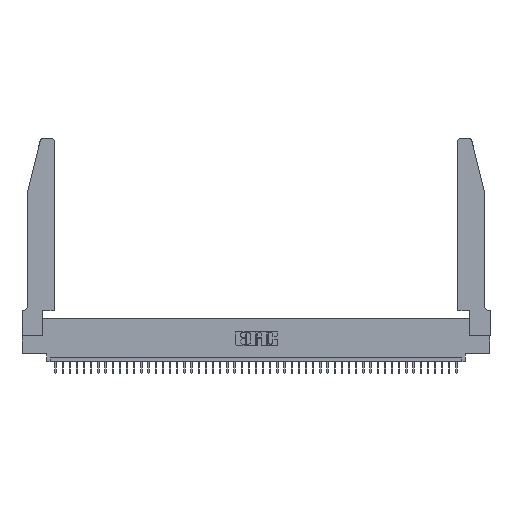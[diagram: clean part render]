
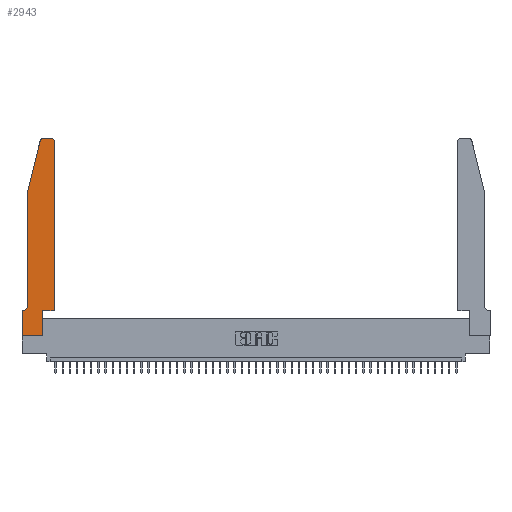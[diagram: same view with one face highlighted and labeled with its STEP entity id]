
A CAD part, top view. The second image highlights one B-rep face of the part: STEP entity #2943.
In plain terms, the highlighted planar face has unit normal (0, 0, 1).
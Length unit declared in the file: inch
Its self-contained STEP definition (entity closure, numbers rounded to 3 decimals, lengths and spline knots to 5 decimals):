
#106 = EDGE_CURVE ( 'NONE', #34860, #22482, #16023, .T. ) ;
#476 = VERTEX_POINT ( 'NONE', #846 ) ;
#504 = CARTESIAN_POINT ( 'NONE',  ( 0.0055, 0.35, 0.37 ) ) ;
#836 = DIRECTION ( 'NONE',  ( 0., 1., 0. ) ) ;
#846 = CARTESIAN_POINT ( 'NONE',  ( 0.4505, 0.35, 0.37 ) ) ;
#949 = LINE ( 'NONE', #4083, #23601 ) ;
#1282 = DIRECTION ( 'NONE',  ( 1., 0., 0. ) ) ;
#1801 = CIRCLE ( 'NONE', #14285, 0.03 ) ;
#1964 = VECTOR ( 'NONE', #4756, 39.37008 ) ;
#2101 = CARTESIAN_POINT ( 'NONE',  ( 0.284, 2.75, 0.37 ) ) ;
#2395 = ORIENTED_EDGE ( 'NONE', *, *, #23045, .T. ) ;
#2943 = ADVANCED_FACE ( 'NONE', ( #12163 ), #3575, .T. ) ;
#3575 = PLANE ( 'NONE',  #34172 ) ;
#4044 = VERTEX_POINT ( 'NONE', #26519 ) ;
#4083 = CARTESIAN_POINT ( 'NONE',  ( 0.4505, 0.35, 0.37 ) ) ;
#4433 = CARTESIAN_POINT ( 'NONE',  ( 0.284, 2.72, 0.37 ) ) ;
#4756 = DIRECTION ( 'NONE',  ( -0.239, -0.971, 0. ) ) ;
#5907 = ORIENTED_EDGE ( 'NONE', *, *, #36275, .T. ) ;
#6338 = VERTEX_POINT ( 'NONE', #42171 ) ;
#6488 = DIRECTION ( 'NONE',  ( -1., 0., 0. ) ) ;
#6923 = CARTESIAN_POINT ( 'NONE',  ( 0., 0., 0.37 ) ) ;
#8188 = EDGE_CURVE ( 'NONE', #476, #33832, #12763, .T. ) ;
#8206 = CARTESIAN_POINT ( 'NONE',  ( 0.2865, 0.35, 0.37 ) ) ;
#9088 = VECTOR ( 'NONE', #36396, 39.37008 ) ;
#9766 = VECTOR ( 'NONE', #41715, 39.37008 ) ;
#11070 = CARTESIAN_POINT ( 'NONE',  ( 0.4205, 2.75, 0.37 ) ) ;
#11316 = VERTEX_POINT ( 'NONE', #11070 ) ;
#11942 = VERTEX_POINT ( 'NONE', #45766 ) ;
#12163 = FACE_OUTER_BOUND ( 'NONE', #22378, .T. ) ;
#12361 = VECTOR ( 'NONE', #15133, 39.37008 ) ;
#12508 = DIRECTION ( 'NONE',  ( 0., 0., -1. ) ) ;
#12763 = LINE ( 'NONE', #30459, #39845 ) ;
#13583 = CARTESIAN_POINT ( 'NONE',  ( 0.2605, 2.75, 0.37 ) ) ;
#14285 = AXIS2_PLACEMENT_3D ( 'NONE', #4433, #32715, #39674 ) ;
#14434 = LINE ( 'NONE', #6923, #39282 ) ;
#15133 = DIRECTION ( 'NONE',  ( 0., -1., 0. ) ) ;
#15199 = DIRECTION ( 'NONE',  ( 0., 0., 1. ) ) ;
#15929 = CARTESIAN_POINT ( 'NONE',  ( 0.0755, 2., 0.37 ) ) ;
#16023 = LINE ( 'NONE', #22967, #24297 ) ;
#16183 = AXIS2_PLACEMENT_3D ( 'NONE', #33797, #12508, #6488 ) ;
#17705 = DIRECTION ( 'NONE',  ( 1., 0., 0. ) ) ;
#18734 = EDGE_CURVE ( 'NONE', #33832, #11316, #38677, .T. ) ;
#18777 = CARTESIAN_POINT ( 'NONE',  ( 0., 0.35, 0.37 ) ) ;
#20297 = AXIS2_PLACEMENT_3D ( 'NONE', #29081, #15199, #1282 ) ;
#22378 = EDGE_LOOP ( 'NONE', ( #26464, #5907, #39334, #33928, #29792, #31390, #31758, #31178, #31262, #2395, #26244, #45220 ) ) ;
#22482 = VERTEX_POINT ( 'NONE', #18777 ) ;
#22630 = CARTESIAN_POINT ( 'NONE',  ( 0.0755, 0.42, 0.37 ) ) ;
#22681 = VERTEX_POINT ( 'NONE', #2101 ) ;
#22819 = DIRECTION ( 'NONE',  ( -1., 0., 0. ) ) ;
#22967 = CARTESIAN_POINT ( 'NONE',  ( 0.0755, 0.35, 0.37 ) ) ;
#23045 = EDGE_CURVE ( 'NONE', #27252, #476, #949, .T. ) ;
#23601 = VECTOR ( 'NONE', #43363, 39.37008 ) ;
#24297 = VECTOR ( 'NONE', #22819, 39.37008 ) ;
#24452 = EDGE_CURVE ( 'NONE', #22482, #6338, #45661, .T. ) ;
#25038 = DIRECTION ( 'NONE',  ( 0., 0., 1. ) ) ;
#25108 = CARTESIAN_POINT ( 'NONE',  ( 0.0755, 2., 0.37 ) ) ;
#26122 = VECTOR ( 'NONE', #836, 39.37008 ) ;
#26244 = ORIENTED_EDGE ( 'NONE', *, *, #8188, .T. ) ;
#26464 = ORIENTED_EDGE ( 'NONE', *, *, #28645, .T. ) ;
#26519 = CARTESIAN_POINT ( 'NONE',  ( 0.25487, 2.72718, 0.37 ) ) ;
#26900 = EDGE_CURVE ( 'NONE', #6338, #11942, #14434, .T. ) ;
#27252 = VERTEX_POINT ( 'NONE', #8206 ) ;
#28302 = CARTESIAN_POINT ( 'NONE',  ( 0., 0.35, 0.37 ) ) ;
#28645 = EDGE_CURVE ( 'NONE', #11316, #22681, #35145, .T. ) ;
#28865 = CARTESIAN_POINT ( 'NONE',  ( 0.0755, 2., 0.37 ) ) ;
#28924 = CARTESIAN_POINT ( 'NONE',  ( 0.2865, 0.35, 0.37 ) ) ;
#28969 = EDGE_CURVE ( 'NONE', #4044, #34662, #41794, .T. ) ;
#29081 = CARTESIAN_POINT ( 'NONE',  ( 0.4205, 2.72, 0.37 ) ) ;
#29151 = VERTEX_POINT ( 'NONE', #22630 ) ;
#29792 = ORIENTED_EDGE ( 'NONE', *, *, #29945, .T. ) ;
#29945 = EDGE_CURVE ( 'NONE', #29151, #34860, #30689, .T. ) ;
#30459 = CARTESIAN_POINT ( 'NONE',  ( 0.4505, 0.35, 0.37 ) ) ;
#30689 = CIRCLE ( 'NONE', #16183, 0.07 ) ;
#31086 = LINE ( 'NONE', #28924, #26122 ) ;
#31163 = LINE ( 'NONE', #28865, #12361 ) ;
#31178 = ORIENTED_EDGE ( 'NONE', *, *, #26900, .T. ) ;
#31262 = ORIENTED_EDGE ( 'NONE', *, *, #39937, .T. ) ;
#31390 = ORIENTED_EDGE ( 'NONE', *, *, #106, .T. ) ;
#31405 = CARTESIAN_POINT ( 'NONE',  ( 0., 0., 0.37 ) ) ;
#31758 = ORIENTED_EDGE ( 'NONE', *, *, #24452, .T. ) ;
#32715 = DIRECTION ( 'NONE',  ( 0., 0., 1. ) ) ;
#33797 = CARTESIAN_POINT ( 'NONE',  ( 0.0055, 0.42, 0.37 ) ) ;
#33832 = VERTEX_POINT ( 'NONE', #36196 ) ;
#33928 = ORIENTED_EDGE ( 'NONE', *, *, #45568, .T. ) ;
#34172 = AXIS2_PLACEMENT_3D ( 'NONE', #28302, #25038, #39396 ) ;
#34662 = VERTEX_POINT ( 'NONE', #25108 ) ;
#34860 = VERTEX_POINT ( 'NONE', #504 ) ;
#35145 = LINE ( 'NONE', #13583, #9766 ) ;
#36196 = CARTESIAN_POINT ( 'NONE',  ( 0.4505, 2.72, 0.37 ) ) ;
#36275 = EDGE_CURVE ( 'NONE', #22681, #4044, #1801, .T. ) ;
#36396 = DIRECTION ( 'NONE',  ( 0., -1., 0. ) ) ;
#38677 = CIRCLE ( 'NONE', #20297, 0.03 ) ;
#39282 = VECTOR ( 'NONE', #17705, 39.37008 ) ;
#39334 = ORIENTED_EDGE ( 'NONE', *, *, #28969, .T. ) ;
#39396 = DIRECTION ( 'NONE',  ( 1., 0., 0. ) ) ;
#39674 = DIRECTION ( 'NONE',  ( 1., 0., 0. ) ) ;
#39845 = VECTOR ( 'NONE', #44419, 39.37008 ) ;
#39937 = EDGE_CURVE ( 'NONE', #11942, #27252, #31086, .T. ) ;
#41715 = DIRECTION ( 'NONE',  ( -1., 0., 0. ) ) ;
#41794 = LINE ( 'NONE', #15929, #1964 ) ;
#42171 = CARTESIAN_POINT ( 'NONE',  ( 0., 0., 0.37 ) ) ;
#43363 = DIRECTION ( 'NONE',  ( 1., 0., 0. ) ) ;
#44419 = DIRECTION ( 'NONE',  ( 0., 1., 0. ) ) ;
#45220 = ORIENTED_EDGE ( 'NONE', *, *, #18734, .T. ) ;
#45568 = EDGE_CURVE ( 'NONE', #34662, #29151, #31163, .T. ) ;
#45661 = LINE ( 'NONE', #31405, #9088 ) ;
#45766 = CARTESIAN_POINT ( 'NONE',  ( 0.2865, 0., 0.37 ) ) ;
